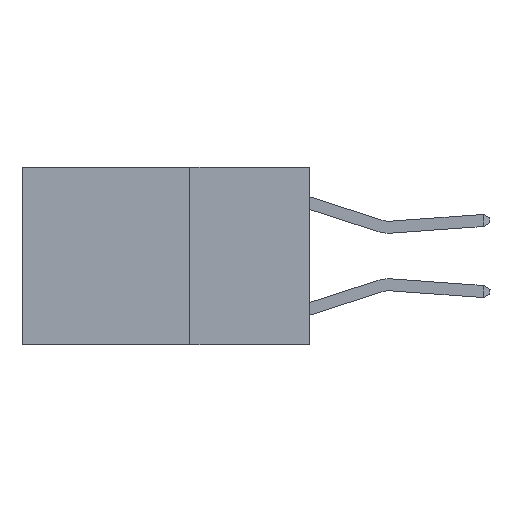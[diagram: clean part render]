
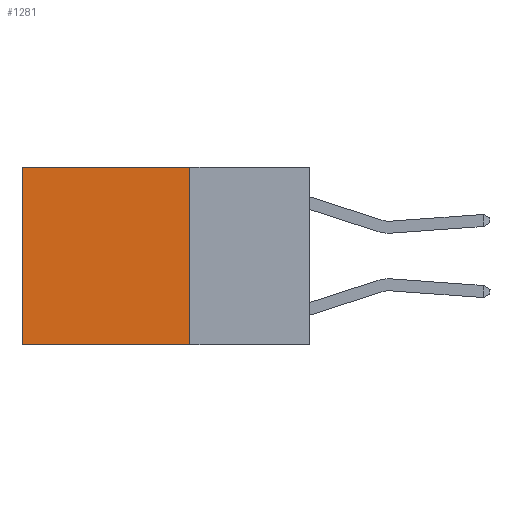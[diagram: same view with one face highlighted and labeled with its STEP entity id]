
A CAD part, left-side view. The second image highlights one B-rep face of the part: STEP entity #1281.
In plain terms, the highlighted planar face has unit normal (-1, 0, 0).
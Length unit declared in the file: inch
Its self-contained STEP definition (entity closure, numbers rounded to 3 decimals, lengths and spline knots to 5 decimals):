
#1049 = VERTEX_POINT ( 'NONE', #20796 ) ;
#1281 = ADVANCED_FACE ( 'NONE', ( #16929 ), #10457, .F. ) ;
#1811 = VECTOR ( 'NONE', #19005, 39.37008 ) ;
#1947 = DIRECTION ( 'NONE',  ( 0., 1., 0. ) ) ;
#2807 = LINE ( 'NONE', #23447, #11930 ) ;
#3886 = LINE ( 'NONE', #8165, #1811 ) ;
#5105 = ORIENTED_EDGE ( 'NONE', *, *, #17881, .T. ) ;
#7342 = VERTEX_POINT ( 'NONE', #17785 ) ;
#8165 = CARTESIAN_POINT ( 'NONE',  ( 0.2625, 0.6, 0. ) ) ;
#10457 = PLANE ( 'NONE',  #23759 ) ;
#10787 = EDGE_LOOP ( 'NONE', ( #15745, #11606, #13298, #5105 ) ) ;
#11204 = DIRECTION ( 'NONE',  ( 0., 0., -1. ) ) ;
#11540 = DIRECTION ( 'NONE',  ( 0., 1., 0. ) ) ;
#11606 = ORIENTED_EDGE ( 'NONE', *, *, #12444, .F. ) ;
#11930 = VECTOR ( 'NONE', #11204, 39.37008 ) ;
#12444 = EDGE_CURVE ( 'NONE', #7342, #21584, #20792, .T. ) ;
#12735 = CARTESIAN_POINT ( 'NONE',  ( 0.2625, 0.25, 0. ) ) ;
#13298 = ORIENTED_EDGE ( 'NONE', *, *, #20162, .F. ) ;
#14316 = VERTEX_POINT ( 'NONE', #12735 ) ;
#15745 = ORIENTED_EDGE ( 'NONE', *, *, #20412, .T. ) ;
#16255 = VECTOR ( 'NONE', #1947, 39.37008 ) ;
#16929 = FACE_OUTER_BOUND ( 'NONE', #10787, .T. ) ;
#17609 = DIRECTION ( 'NONE',  ( 0., 0., -1. ) ) ;
#17785 = CARTESIAN_POINT ( 'NONE',  ( 0.2625, 0.25, -0.37 ) ) ;
#17881 = EDGE_CURVE ( 'NONE', #14316, #1049, #26097, .T. ) ;
#18853 = DIRECTION ( 'NONE',  ( 1., 0., 0. ) ) ;
#19005 = DIRECTION ( 'NONE',  ( 0., 0., -1. ) ) ;
#20162 = EDGE_CURVE ( 'NONE', #14316, #7342, #2807, .T. ) ;
#20412 = EDGE_CURVE ( 'NONE', #1049, #21584, #3886, .T. ) ;
#20792 = LINE ( 'NONE', #26684, #16255 ) ;
#20796 = CARTESIAN_POINT ( 'NONE',  ( 0.2625, 0.6, 0. ) ) ;
#21584 = VERTEX_POINT ( 'NONE', #21798 ) ;
#21798 = CARTESIAN_POINT ( 'NONE',  ( 0.2625, 0.6, -0.37 ) ) ;
#23447 = CARTESIAN_POINT ( 'NONE',  ( 0.2625, 0.25, 0. ) ) ;
#23759 = AXIS2_PLACEMENT_3D ( 'NONE', #25293, #18853, #17609 ) ;
#25293 = CARTESIAN_POINT ( 'NONE',  ( 0.2625, 0.25, 0. ) ) ;
#25491 = VECTOR ( 'NONE', #11540, 39.37008 ) ;
#25814 = CARTESIAN_POINT ( 'NONE',  ( 0.2625, 0.25, 0. ) ) ;
#26097 = LINE ( 'NONE', #25814, #25491 ) ;
#26684 = CARTESIAN_POINT ( 'NONE',  ( 0.2625, 0.25, -0.37 ) ) ;
